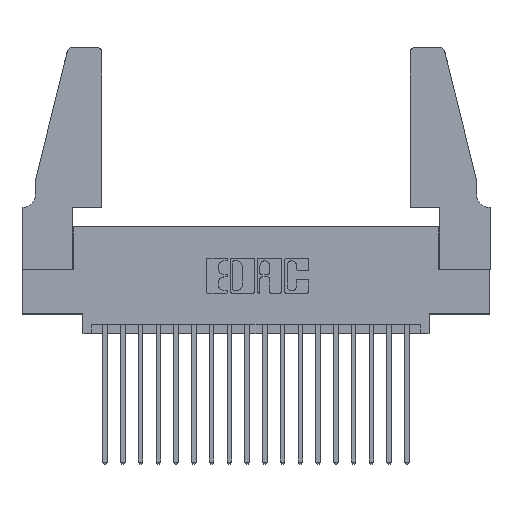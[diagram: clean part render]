
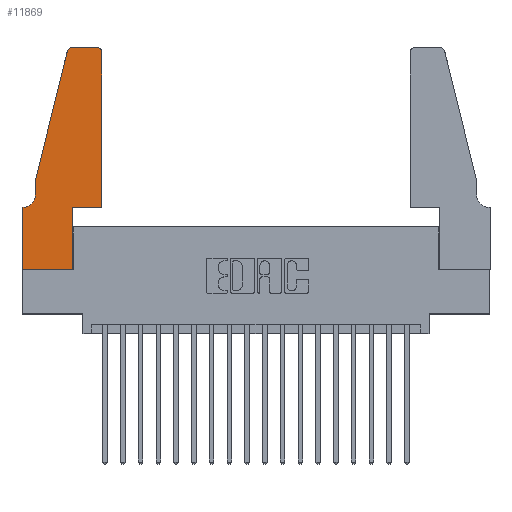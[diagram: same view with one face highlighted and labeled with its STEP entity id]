
A CAD part, top view. The second image highlights one B-rep face of the part: STEP entity #11869.
In plain terms, the highlighted planar face has unit normal (0, 0, 1).
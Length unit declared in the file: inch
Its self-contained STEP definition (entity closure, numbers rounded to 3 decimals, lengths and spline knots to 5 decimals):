
#107 = LINE ( 'NONE', #6160, #16748 ) ;
#348 = DIRECTION ( 'NONE',  ( 0., 0., 1. ) ) ;
#394 = DIRECTION ( 'NONE',  ( 1., 0., 0. ) ) ;
#413 = PLANE ( 'NONE',  #9712 ) ;
#572 = VERTEX_POINT ( 'NONE', #16326 ) ;
#634 = LINE ( 'NONE', #10848, #1359 ) ;
#811 = CARTESIAN_POINT ( 'NONE',  ( 0.2865, 0., 0.37 ) ) ;
#999 = CARTESIAN_POINT ( 'NONE',  ( 0.4505, 1.22, 0.37 ) ) ;
#1041 = EDGE_CURVE ( 'NONE', #13097, #14891, #10979, .T. ) ;
#1140 = LINE ( 'NONE', #3273, #14468 ) ;
#1314 = VERTEX_POINT ( 'NONE', #3914 ) ;
#1359 = VECTOR ( 'NONE', #394, 39.37008 ) ;
#1758 = ORIENTED_EDGE ( 'NONE', *, *, #7447, .T. ) ;
#1885 = VERTEX_POINT ( 'NONE', #6315 ) ;
#1951 = EDGE_CURVE ( 'NONE', #17088, #572, #3265, .T. ) ;
#2643 = EDGE_CURVE ( 'NONE', #1885, #13097, #634, .T. ) ;
#2822 = VERTEX_POINT ( 'NONE', #999 ) ;
#2975 = CIRCLE ( 'NONE', #13113, 0.07 ) ;
#3123 = DIRECTION ( 'NONE',  ( -1., 0., 0. ) ) ;
#3265 = LINE ( 'NONE', #4990, #8719 ) ;
#3272 = CARTESIAN_POINT ( 'NONE',  ( 0.0055, 0.42, 0.37 ) ) ;
#3273 = CARTESIAN_POINT ( 'NONE',  ( 0.0755, 0.35, 0.37 ) ) ;
#3406 = ORIENTED_EDGE ( 'NONE', *, *, #9879, .T. ) ;
#3677 = EDGE_CURVE ( 'NONE', #15876, #2822, #7209, .T. ) ;
#3910 = EDGE_CURVE ( 'NONE', #18614, #5792, #2975, .T. ) ;
#3914 = CARTESIAN_POINT ( 'NONE',  ( 0.4205, 1.25, 0.37 ) ) ;
#4320 = DIRECTION ( 'NONE',  ( 0., 1., 0. ) ) ;
#4816 = DIRECTION ( 'NONE',  ( -1., 0., 0. ) ) ;
#4919 = CARTESIAN_POINT ( 'NONE',  ( 0.4505, 0.35, 0.37 ) ) ;
#4990 = CARTESIAN_POINT ( 'NONE',  ( 0.0755, 0.5, 0.37 ) ) ;
#5380 = DIRECTION ( 'NONE',  ( -0.239, -0.971, 0. ) ) ;
#5448 = CARTESIAN_POINT ( 'NONE',  ( 0.25487, 1.22718, 0.37 ) ) ;
#5499 = DIRECTION ( 'NONE',  ( 0., 0., 1. ) ) ;
#5628 = FACE_OUTER_BOUND ( 'NONE', #14194, .T. ) ;
#5695 = CARTESIAN_POINT ( 'NONE',  ( 0.4205, 1.22, 0.37 ) ) ;
#5792 = VERTEX_POINT ( 'NONE', #13906 ) ;
#5800 = ORIENTED_EDGE ( 'NONE', *, *, #2643, .T. ) ;
#5935 = VECTOR ( 'NONE', #13249, 39.37008 ) ;
#6160 = CARTESIAN_POINT ( 'NONE',  ( 0.2605, 1.25, 0.37 ) ) ;
#6290 = CARTESIAN_POINT ( 'NONE',  ( 0.0755, 0.5, 0.37 ) ) ;
#6309 = DIRECTION ( 'NONE',  ( 0., 1., 0. ) ) ;
#6315 = CARTESIAN_POINT ( 'NONE',  ( 0., 0., 0.37 ) ) ;
#7057 = LINE ( 'NONE', #17819, #5935 ) ;
#7209 = LINE ( 'NONE', #4919, #19394 ) ;
#7447 = EDGE_CURVE ( 'NONE', #5792, #19410, #1140, .T. ) ;
#7472 = VECTOR ( 'NONE', #13461, 39.37008 ) ;
#7934 = CARTESIAN_POINT ( 'NONE',  ( 0., 0.35, 0.37 ) ) ;
#8719 = VECTOR ( 'NONE', #5380, 39.37008 ) ;
#8725 = VERTEX_POINT ( 'NONE', #19017 ) ;
#8850 = ORIENTED_EDGE ( 'NONE', *, *, #17611, .T. ) ;
#8942 = CARTESIAN_POINT ( 'NONE',  ( 0., 0.35, 0.37 ) ) ;
#9538 = ORIENTED_EDGE ( 'NONE', *, *, #3677, .T. ) ;
#9712 = AXIS2_PLACEMENT_3D ( 'NONE', #7934, #348, #14062 ) ;
#9879 = EDGE_CURVE ( 'NONE', #8725, #17088, #10464, .T. ) ;
#10102 = EDGE_CURVE ( 'NONE', #19410, #1885, #7057, .T. ) ;
#10163 = ORIENTED_EDGE ( 'NONE', *, *, #19636, .T. ) ;
#10263 = ORIENTED_EDGE ( 'NONE', *, *, #12101, .T. ) ;
#10398 = CARTESIAN_POINT ( 'NONE',  ( 0.2865, 0.35, 0.37 ) ) ;
#10458 = ORIENTED_EDGE ( 'NONE', *, *, #1041, .T. ) ;
#10464 = CIRCLE ( 'NONE', #19550, 0.03 ) ;
#10848 = CARTESIAN_POINT ( 'NONE',  ( 0., 0., 0.37 ) ) ;
#10911 = DIRECTION ( 'NONE',  ( 0., -1., 0. ) ) ;
#10979 = LINE ( 'NONE', #10398, #14084 ) ;
#11362 = CARTESIAN_POINT ( 'NONE',  ( 0.4505, 0.35, 0.37 ) ) ;
#11869 = ADVANCED_FACE ( 'NONE', ( #5628 ), #413, .T. ) ;
#12062 = ORIENTED_EDGE ( 'NONE', *, *, #12731, .T. ) ;
#12101 = EDGE_CURVE ( 'NONE', #2822, #1314, #18481, .T. ) ;
#12192 = AXIS2_PLACEMENT_3D ( 'NONE', #5695, #5499, #16216 ) ;
#12245 = DIRECTION ( 'NONE',  ( -1., 0., 0. ) ) ;
#12359 = ORIENTED_EDGE ( 'NONE', *, *, #10102, .T. ) ;
#12731 = EDGE_CURVE ( 'NONE', #14891, #15876, #16567, .T. ) ;
#13097 = VERTEX_POINT ( 'NONE', #811 ) ;
#13113 = AXIS2_PLACEMENT_3D ( 'NONE', #3272, #16607, #3123 ) ;
#13249 = DIRECTION ( 'NONE',  ( 0., -1., 0. ) ) ;
#13461 = DIRECTION ( 'NONE',  ( 1., 0., 0. ) ) ;
#13906 = CARTESIAN_POINT ( 'NONE',  ( 0.0055, 0.35, 0.37 ) ) ;
#14062 = DIRECTION ( 'NONE',  ( 1., 0., 0. ) ) ;
#14084 = VECTOR ( 'NONE', #4320, 39.37008 ) ;
#14194 = EDGE_LOOP ( 'NONE', ( #10163, #3406, #18731, #8850, #14616, #1758, #12359, #5800, #10458, #12062, #9538, #10263 ) ) ;
#14468 = VECTOR ( 'NONE', #4816, 39.37008 ) ;
#14616 = ORIENTED_EDGE ( 'NONE', *, *, #3910, .T. ) ;
#14891 = VERTEX_POINT ( 'NONE', #16994 ) ;
#15820 = LINE ( 'NONE', #6290, #18447 ) ;
#15876 = VERTEX_POINT ( 'NONE', #11362 ) ;
#16216 = DIRECTION ( 'NONE',  ( 1., 0., 0. ) ) ;
#16244 = CARTESIAN_POINT ( 'NONE',  ( 0.0755, 0.42, 0.37 ) ) ;
#16326 = CARTESIAN_POINT ( 'NONE',  ( 0.0755, 0.5, 0.37 ) ) ;
#16567 = LINE ( 'NONE', #17825, #7472 ) ;
#16607 = DIRECTION ( 'NONE',  ( 0., 0., -1. ) ) ;
#16748 = VECTOR ( 'NONE', #12245, 39.37008 ) ;
#16994 = CARTESIAN_POINT ( 'NONE',  ( 0.2865, 0.35, 0.37 ) ) ;
#17088 = VERTEX_POINT ( 'NONE', #5448 ) ;
#17237 = DIRECTION ( 'NONE',  ( 1., 0., 0. ) ) ;
#17611 = EDGE_CURVE ( 'NONE', #572, #18614, #15820, .T. ) ;
#17819 = CARTESIAN_POINT ( 'NONE',  ( 0., 0., 0.37 ) ) ;
#17825 = CARTESIAN_POINT ( 'NONE',  ( 0.4505, 0.35, 0.37 ) ) ;
#18447 = VECTOR ( 'NONE', #10911, 39.37008 ) ;
#18481 = CIRCLE ( 'NONE', #12192, 0.03 ) ;
#18614 = VERTEX_POINT ( 'NONE', #16244 ) ;
#18627 = CARTESIAN_POINT ( 'NONE',  ( 0.284, 1.22, 0.37 ) ) ;
#18731 = ORIENTED_EDGE ( 'NONE', *, *, #1951, .T. ) ;
#18748 = DIRECTION ( 'NONE',  ( 0., 0., 1. ) ) ;
#19017 = CARTESIAN_POINT ( 'NONE',  ( 0.284, 1.25, 0.37 ) ) ;
#19394 = VECTOR ( 'NONE', #6309, 39.37008 ) ;
#19410 = VERTEX_POINT ( 'NONE', #8942 ) ;
#19550 = AXIS2_PLACEMENT_3D ( 'NONE', #18627, #18748, #17237 ) ;
#19636 = EDGE_CURVE ( 'NONE', #1314, #8725, #107, .T. ) ;
